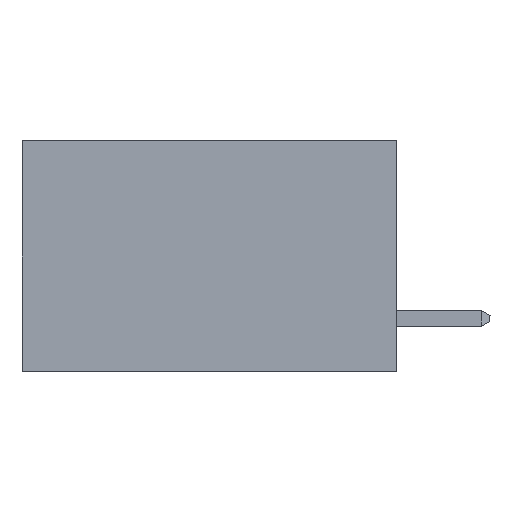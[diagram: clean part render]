
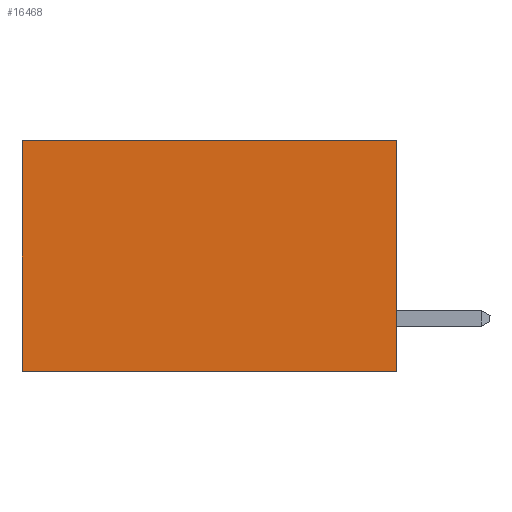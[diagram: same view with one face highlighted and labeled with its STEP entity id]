
A CAD part, left-side view. The second image highlights one B-rep face of the part: STEP entity #16468.
In plain terms, the highlighted planar face has unit normal (-1, 0, 0).
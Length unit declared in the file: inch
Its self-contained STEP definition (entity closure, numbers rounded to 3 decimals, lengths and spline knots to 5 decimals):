
#532 = VERTEX_POINT ( 'NONE', #10250 ) ;
#543 = CARTESIAN_POINT ( 'NONE',  ( 0.2615, 0., 0. ) ) ;
#694 = CARTESIAN_POINT ( 'NONE',  ( 0.2615, 0., 0. ) ) ;
#1033 = DIRECTION ( 'NONE',  ( 0., 0., -1. ) ) ;
#1643 = CARTESIAN_POINT ( 'NONE',  ( 0.2615, 0., -0.37 ) ) ;
#1875 = EDGE_CURVE ( 'NONE', #5517, #16519, #17522, .T. ) ;
#2398 = CARTESIAN_POINT ( 'NONE',  ( 0.2615, 0.6, 0. ) ) ;
#3467 = CARTESIAN_POINT ( 'NONE',  ( 0.2615, 0., -0.37 ) ) ;
#5420 = VECTOR ( 'NONE', #7346, 39.37008 ) ;
#5437 = DIRECTION ( 'NONE',  ( 0., 0., -1. ) ) ;
#5517 = VERTEX_POINT ( 'NONE', #2398 ) ;
#6474 = ORIENTED_EDGE ( 'NONE', *, *, #1875, .T. ) ;
#7128 = DIRECTION ( 'NONE',  ( 1., 0., 0. ) ) ;
#7346 = DIRECTION ( 'NONE',  ( 0., 1., 0. ) ) ;
#7455 = PLANE ( 'NONE',  #15147 ) ;
#7829 = EDGE_CURVE ( 'NONE', #532, #16519, #11374, .T. ) ;
#8142 = VECTOR ( 'NONE', #5437, 39.37008 ) ;
#9719 = CARTESIAN_POINT ( 'NONE',  ( 0.2615, 0.6, -0.37 ) ) ;
#9722 = EDGE_LOOP ( 'NONE', ( #6474, #9990, #18285, #17681 ) ) ;
#9990 = ORIENTED_EDGE ( 'NONE', *, *, #7829, .F. ) ;
#10250 = CARTESIAN_POINT ( 'NONE',  ( 0.2615, 0., -0.37 ) ) ;
#11191 = VECTOR ( 'NONE', #1033, 39.37008 ) ;
#11374 = LINE ( 'NONE', #1643, #16590 ) ;
#12256 = LINE ( 'NONE', #694, #5420 ) ;
#14110 = CARTESIAN_POINT ( 'NONE',  ( 0.2615, 0., -0.37 ) ) ;
#15147 = AXIS2_PLACEMENT_3D ( 'NONE', #14110, #7128, #20775 ) ;
#15285 = VERTEX_POINT ( 'NONE', #543 ) ;
#15423 = FACE_OUTER_BOUND ( 'NONE', #9722, .T. ) ;
#15542 = EDGE_CURVE ( 'NONE', #15285, #532, #20399, .T. ) ;
#16468 = ADVANCED_FACE ( 'NONE', ( #15423 ), #7455, .F. ) ;
#16519 = VERTEX_POINT ( 'NONE', #9719 ) ;
#16590 = VECTOR ( 'NONE', #19663, 39.37008 ) ;
#17522 = LINE ( 'NONE', #17630, #11191 ) ;
#17630 = CARTESIAN_POINT ( 'NONE',  ( 0.2615, 0.6, -0.37 ) ) ;
#17681 = ORIENTED_EDGE ( 'NONE', *, *, #17792, .T. ) ;
#17792 = EDGE_CURVE ( 'NONE', #15285, #5517, #12256, .T. ) ;
#18285 = ORIENTED_EDGE ( 'NONE', *, *, #15542, .F. ) ;
#19663 = DIRECTION ( 'NONE',  ( 0., 1., 0. ) ) ;
#20399 = LINE ( 'NONE', #3467, #8142 ) ;
#20775 = DIRECTION ( 'NONE',  ( 0., 0., -1. ) ) ;
